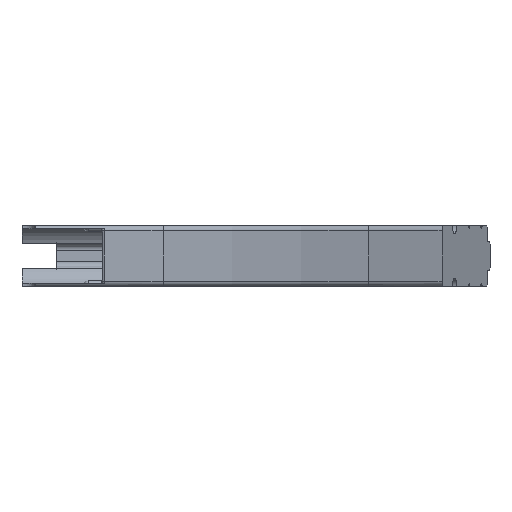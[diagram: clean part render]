
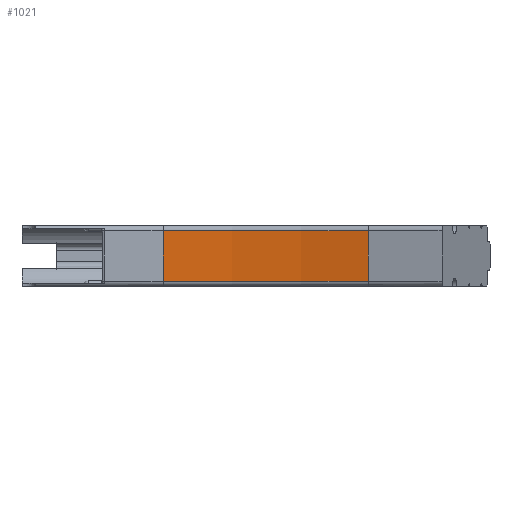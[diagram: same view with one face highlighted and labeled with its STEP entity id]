
A CAD part, left-side view. The second image highlights one B-rep face of the part: STEP entity #1021.
In plain terms, the highlighted cylindrical face has radius 265.821 mm (diameter 531.643 mm), a partial arc.
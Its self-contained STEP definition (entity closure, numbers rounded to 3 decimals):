
#182 = AXIS2_PLACEMENT_3D ( 'NONE', #2518, #1700, #4402 ) ;
#685 = VECTOR ( 'NONE', #1130, 1000. ) ;
#697 = VERTEX_POINT ( 'NONE', #4299 ) ;
#802 = EDGE_CURVE ( 'NONE', #3177, #3551, #3832, .T. ) ;
#812 = FACE_OUTER_BOUND ( 'NONE', #3943, .T. ) ;
#1021 = ADVANCED_FACE ( 'NONE', ( #812 ), #4257, .F. ) ;
#1130 = DIRECTION ( 'NONE',  ( 0., 0., -1. ) ) ;
#1583 = EDGE_CURVE ( 'NONE', #3177, #697, #1718, .T. ) ;
#1700 = DIRECTION ( 'NONE',  ( 0., 0., 1. ) ) ;
#1718 = LINE ( 'NONE', #1888, #685 ) ;
#1888 = CARTESIAN_POINT ( 'NONE',  ( -43.147, -130., 11.4 ) ) ;
#2035 = DIRECTION ( 'NONE',  ( -1., 0., 0. ) ) ;
#2165 = AXIS2_PLACEMENT_3D ( 'NONE', #4860, #2907, #2958 ) ;
#2187 = CARTESIAN_POINT ( 'NONE',  ( -31.75, -53., 9.4 ) ) ;
#2220 = VECTOR ( 'NONE', #2661, 1000. ) ;
#2261 = CARTESIAN_POINT ( 'NONE',  ( -31.75, -53., -9.4 ) ) ;
#2326 = CIRCLE ( 'NONE', #3003, 265.821 ) ;
#2518 = CARTESIAN_POINT ( 'NONE',  ( -297.571, -53., 9.4 ) ) ;
#2661 = DIRECTION ( 'NONE',  ( 0., 0., -1. ) ) ;
#2907 = DIRECTION ( 'NONE',  ( 0., 0., -1. ) ) ;
#2958 = DIRECTION ( 'NONE',  ( -1., 0., 0. ) ) ;
#3003 = AXIS2_PLACEMENT_3D ( 'NONE', #4757, #3559, #2035 ) ;
#3041 = VERTEX_POINT ( 'NONE', #2261 ) ;
#3126 = LINE ( 'NONE', #4587, #2220 ) ;
#3144 = EDGE_CURVE ( 'NONE', #3551, #3041, #3126, .T. ) ;
#3177 = VERTEX_POINT ( 'NONE', #3443 ) ;
#3313 = EDGE_CURVE ( 'NONE', #697, #3041, #2326, .T. ) ;
#3443 = CARTESIAN_POINT ( 'NONE',  ( -43.147, -130., 9.4 ) ) ;
#3551 = VERTEX_POINT ( 'NONE', #2187 ) ;
#3559 = DIRECTION ( 'NONE',  ( 0., 0., 1. ) ) ;
#3832 = CIRCLE ( 'NONE', #182, 265.821 ) ;
#3943 = EDGE_LOOP ( 'NONE', ( #4862, #4973, #4810, #4748 ) ) ;
#4257 = CYLINDRICAL_SURFACE ( 'NONE', #2165, 265.821 ) ;
#4299 = CARTESIAN_POINT ( 'NONE',  ( -43.147, -130., -9.4 ) ) ;
#4402 = DIRECTION ( 'NONE',  ( -1., 0., 0. ) ) ;
#4587 = CARTESIAN_POINT ( 'NONE',  ( -31.75, -53., 11.4 ) ) ;
#4748 = ORIENTED_EDGE ( 'NONE', *, *, #3313, .F. ) ;
#4757 = CARTESIAN_POINT ( 'NONE',  ( -297.571, -53., -9.4 ) ) ;
#4810 = ORIENTED_EDGE ( 'NONE', *, *, #3144, .T. ) ;
#4860 = CARTESIAN_POINT ( 'NONE',  ( -297.571, -53., 11.4 ) ) ;
#4862 = ORIENTED_EDGE ( 'NONE', *, *, #1583, .F. ) ;
#4973 = ORIENTED_EDGE ( 'NONE', *, *, #802, .T. ) ;
